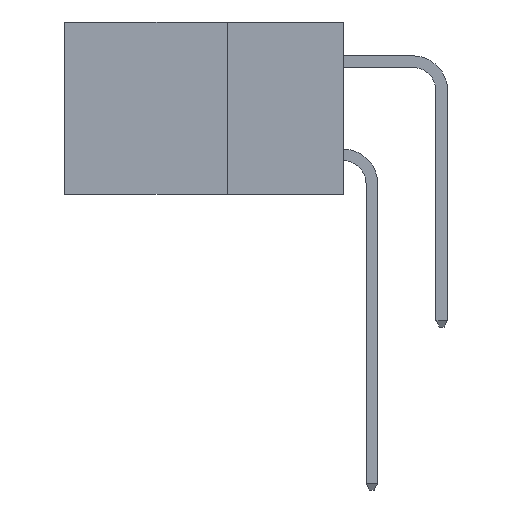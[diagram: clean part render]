
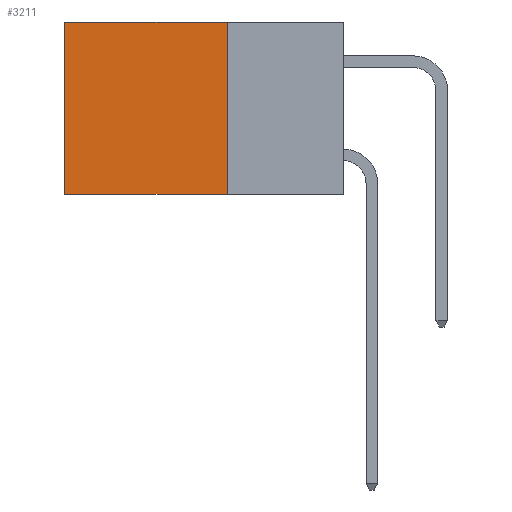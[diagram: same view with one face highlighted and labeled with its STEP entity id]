
A CAD part, left-side view. The second image highlights one B-rep face of the part: STEP entity #3211.
In plain terms, the highlighted planar face has unit normal (-1, 0, 0).
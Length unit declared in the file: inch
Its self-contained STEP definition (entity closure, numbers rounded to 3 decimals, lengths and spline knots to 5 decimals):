
#129 = VERTEX_POINT ( 'NONE', #21025 ) ;
#608 = DIRECTION ( 'NONE',  ( 0., 0., -1. ) ) ;
#1207 = ORIENTED_EDGE ( 'NONE', *, *, #21717, .F. ) ;
#1745 = VECTOR ( 'NONE', #9428, 39.37008 ) ;
#2249 = FACE_OUTER_BOUND ( 'NONE', #15898, .T. ) ;
#2263 = DIRECTION ( 'NONE',  ( 0., 1., 0. ) ) ;
#3211 = ADVANCED_FACE ( 'NONE', ( #2249 ), #17950, .F. ) ;
#3532 = CARTESIAN_POINT ( 'NONE',  ( 0.2615, 0.25, -0.37 ) ) ;
#4066 = ORIENTED_EDGE ( 'NONE', *, *, #4399, .F. ) ;
#4399 = EDGE_CURVE ( 'NONE', #19188, #16313, #21800, .T. ) ;
#4477 = CARTESIAN_POINT ( 'NONE',  ( 0.2615, 0.25, -0.37 ) ) ;
#5779 = AXIS2_PLACEMENT_3D ( 'NONE', #17872, #17765, #17639 ) ;
#5844 = EDGE_CURVE ( 'NONE', #15132, #16313, #7075, .T. ) ;
#6511 = VECTOR ( 'NONE', #17084, 39.37008 ) ;
#7075 = LINE ( 'NONE', #11718, #6511 ) ;
#7227 = LINE ( 'NONE', #16555, #1745 ) ;
#9428 = DIRECTION ( 'NONE',  ( 0., 1., 0. ) ) ;
#9591 = CARTESIAN_POINT ( 'NONE',  ( 0.2615, 0.6, 0. ) ) ;
#9957 = ORIENTED_EDGE ( 'NONE', *, *, #18361, .T. ) ;
#11718 = CARTESIAN_POINT ( 'NONE',  ( 0.2615, 0.6, -0.37 ) ) ;
#12863 = CARTESIAN_POINT ( 'NONE',  ( 0.2615, 0.6, -0.37 ) ) ;
#13748 = ORIENTED_EDGE ( 'NONE', *, *, #5844, .T. ) ;
#15132 = VERTEX_POINT ( 'NONE', #9591 ) ;
#15898 = EDGE_LOOP ( 'NONE', ( #13748, #4066, #1207, #9957 ) ) ;
#16313 = VERTEX_POINT ( 'NONE', #12863 ) ;
#16555 = CARTESIAN_POINT ( 'NONE',  ( 0.2615, 0.25, 0. ) ) ;
#16563 = VECTOR ( 'NONE', #608, 39.37008 ) ;
#16726 = CARTESIAN_POINT ( 'NONE',  ( 0.2615, 0.25, -0.37 ) ) ;
#17084 = DIRECTION ( 'NONE',  ( 0., 0., -1. ) ) ;
#17119 = LINE ( 'NONE', #16726, #16563 ) ;
#17639 = DIRECTION ( 'NONE',  ( 0., 0., -1. ) ) ;
#17765 = DIRECTION ( 'NONE',  ( 1., 0., 0. ) ) ;
#17872 = CARTESIAN_POINT ( 'NONE',  ( 0.2615, 0.25, -0.37 ) ) ;
#17950 = PLANE ( 'NONE',  #5779 ) ;
#18361 = EDGE_CURVE ( 'NONE', #129, #15132, #7227, .T. ) ;
#19188 = VERTEX_POINT ( 'NONE', #4477 ) ;
#21025 = CARTESIAN_POINT ( 'NONE',  ( 0.2615, 0.25, 0. ) ) ;
#21243 = VECTOR ( 'NONE', #2263, 39.37008 ) ;
#21717 = EDGE_CURVE ( 'NONE', #129, #19188, #17119, .T. ) ;
#21800 = LINE ( 'NONE', #3532, #21243 ) ;
